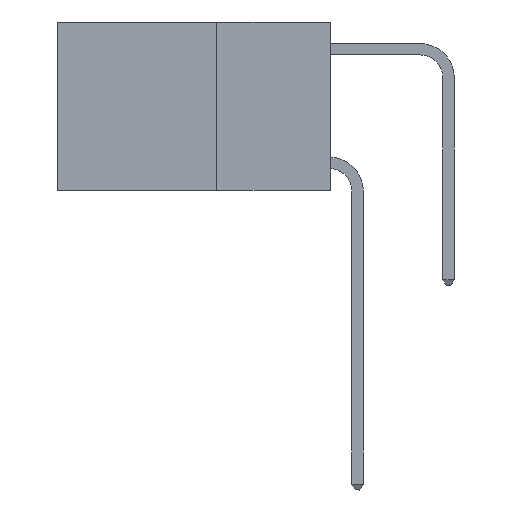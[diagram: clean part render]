
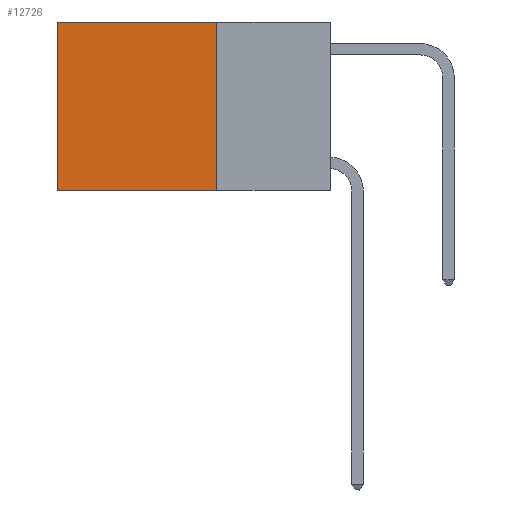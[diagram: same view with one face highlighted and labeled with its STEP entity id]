
A CAD part, left-side view. The second image highlights one B-rep face of the part: STEP entity #12726.
In plain terms, the highlighted planar face has unit normal (-1, 0, 0).
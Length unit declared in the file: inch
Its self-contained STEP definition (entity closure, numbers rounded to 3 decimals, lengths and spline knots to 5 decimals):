
#202 = VERTEX_POINT ( 'NONE', #4079 ) ;
#432 = VERTEX_POINT ( 'NONE', #11501 ) ;
#718 = DIRECTION ( 'NONE',  ( 0., 1., 0. ) ) ;
#1366 = CARTESIAN_POINT ( 'NONE',  ( 0.2625, 0.6, 0. ) ) ;
#1610 = CARTESIAN_POINT ( 'NONE',  ( 0.2625, 0.25, 0. ) ) ;
#1932 = VERTEX_POINT ( 'NONE', #1366 ) ;
#2582 = PLANE ( 'NONE',  #5085 ) ;
#2881 = CARTESIAN_POINT ( 'NONE',  ( 0.2625, 0.6, 0. ) ) ;
#3135 = EDGE_CURVE ( 'NONE', #5753, #1932, #12784, .T. ) ;
#3572 = DIRECTION ( 'NONE',  ( 0., 0., -1. ) ) ;
#4079 = CARTESIAN_POINT ( 'NONE',  ( 0.2625, 0.25, -0.37 ) ) ;
#4127 = DIRECTION ( 'NONE',  ( 0., 1., 0. ) ) ;
#4598 = CARTESIAN_POINT ( 'NONE',  ( 0.2625, 0.25, 0. ) ) ;
#5085 = AXIS2_PLACEMENT_3D ( 'NONE', #4598, #5634, #3572 ) ;
#5154 = DIRECTION ( 'NONE',  ( 0., 0., -1. ) ) ;
#5634 = DIRECTION ( 'NONE',  ( 1., 0., 0. ) ) ;
#5657 = LINE ( 'NONE', #2881, #6272 ) ;
#5753 = VERTEX_POINT ( 'NONE', #8506 ) ;
#6065 = ORIENTED_EDGE ( 'NONE', *, *, #10083, .T. ) ;
#6171 = FACE_OUTER_BOUND ( 'NONE', #11228, .T. ) ;
#6187 = ORIENTED_EDGE ( 'NONE', *, *, #6992, .F. ) ;
#6272 = VECTOR ( 'NONE', #5154, 39.37008 ) ;
#6992 = EDGE_CURVE ( 'NONE', #202, #432, #8051, .T. ) ;
#7326 = ORIENTED_EDGE ( 'NONE', *, *, #8488, .F. ) ;
#7496 = DIRECTION ( 'NONE',  ( 0., 0., -1. ) ) ;
#7582 = VECTOR ( 'NONE', #718, 39.37008 ) ;
#8051 = LINE ( 'NONE', #12112, #7582 ) ;
#8488 = EDGE_CURVE ( 'NONE', #5753, #202, #9640, .T. ) ;
#8506 = CARTESIAN_POINT ( 'NONE',  ( 0.2625, 0.25, 0. ) ) ;
#9640 = LINE ( 'NONE', #1610, #11240 ) ;
#9694 = VECTOR ( 'NONE', #4127, 39.37008 ) ;
#10083 = EDGE_CURVE ( 'NONE', #1932, #432, #5657, .T. ) ;
#11228 = EDGE_LOOP ( 'NONE', ( #6065, #6187, #7326, #12901 ) ) ;
#11240 = VECTOR ( 'NONE', #7496, 39.37008 ) ;
#11501 = CARTESIAN_POINT ( 'NONE',  ( 0.2625, 0.6, -0.37 ) ) ;
#12112 = CARTESIAN_POINT ( 'NONE',  ( 0.2625, 0.25, -0.37 ) ) ;
#12332 = CARTESIAN_POINT ( 'NONE',  ( 0.2625, 0.25, 0. ) ) ;
#12726 = ADVANCED_FACE ( 'NONE', ( #6171 ), #2582, .F. ) ;
#12784 = LINE ( 'NONE', #12332, #9694 ) ;
#12901 = ORIENTED_EDGE ( 'NONE', *, *, #3135, .T. ) ;
